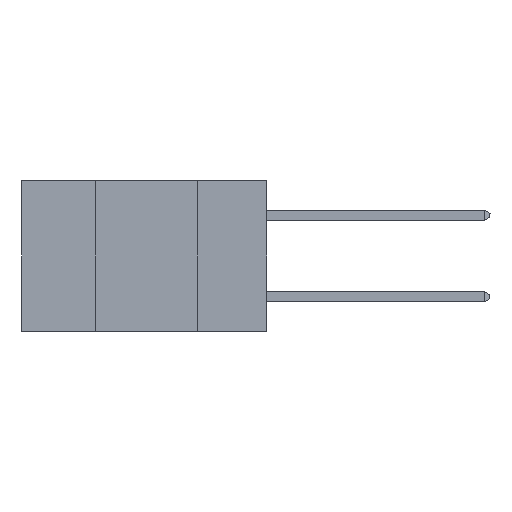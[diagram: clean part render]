
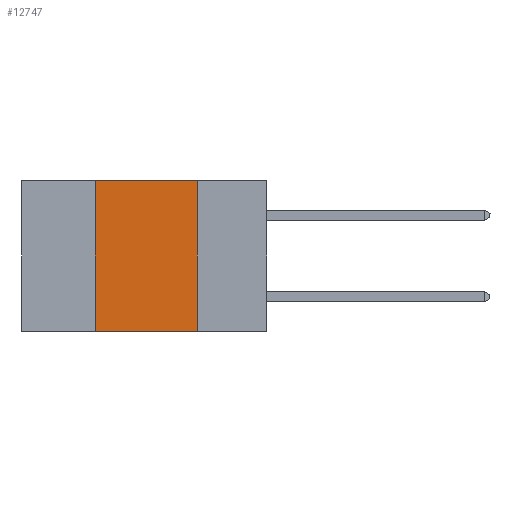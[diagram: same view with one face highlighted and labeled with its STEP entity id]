
A CAD part, left-side view. The second image highlights one B-rep face of the part: STEP entity #12747.
In plain terms, the highlighted planar face has unit normal (-1, 0, 0).
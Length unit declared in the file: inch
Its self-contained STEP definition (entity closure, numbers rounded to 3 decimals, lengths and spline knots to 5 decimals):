
#1166 = LINE ( 'NONE', #14501, #16685 ) ;
#1352 = VECTOR ( 'NONE', #8706, 39.37008 ) ;
#2403 = VECTOR ( 'NONE', #17353, 39.37008 ) ;
#2747 = CARTESIAN_POINT ( 'NONE',  ( 0., 0.17, -0.37 ) ) ;
#3363 = EDGE_CURVE ( 'NONE', #10328, #10754, #1166, .T. ) ;
#4320 = ORIENTED_EDGE ( 'NONE', *, *, #12723, .F. ) ;
#4493 = CARTESIAN_POINT ( 'NONE',  ( 0., 0.6, -0.37 ) ) ;
#5658 = ORIENTED_EDGE ( 'NONE', *, *, #3363, .F. ) ;
#6426 = LINE ( 'NONE', #15829, #2403 ) ;
#7304 = CARTESIAN_POINT ( 'NONE',  ( 0., 0.42, 0. ) ) ;
#7548 = EDGE_LOOP ( 'NONE', ( #5658, #15466, #4320, #10733 ) ) ;
#7818 = VECTOR ( 'NONE', #13415, 39.37008 ) ;
#7916 = CARTESIAN_POINT ( 'NONE',  ( 0., 0.17, 0. ) ) ;
#8090 = DIRECTION ( 'NONE',  ( 0., 0., -1. ) ) ;
#8643 = DIRECTION ( 'NONE',  ( 1., 0., 0. ) ) ;
#8706 = DIRECTION ( 'NONE',  ( 0., -1., 0. ) ) ;
#8777 = CARTESIAN_POINT ( 'NONE',  ( 0., 0.6, 0. ) ) ;
#8998 = CARTESIAN_POINT ( 'NONE',  ( 0., 0.42, -0.37 ) ) ;
#9644 = EDGE_CURVE ( 'NONE', #9987, #10754, #14302, .T. ) ;
#9987 = VERTEX_POINT ( 'NONE', #8998 ) ;
#10328 = VERTEX_POINT ( 'NONE', #7916 ) ;
#10733 = ORIENTED_EDGE ( 'NONE', *, *, #9644, .T. ) ;
#10754 = VERTEX_POINT ( 'NONE', #2747 ) ;
#11597 = FACE_OUTER_BOUND ( 'NONE', #7548, .T. ) ;
#12723 = EDGE_CURVE ( 'NONE', #9987, #15810, #6426, .T. ) ;
#12747 = ADVANCED_FACE ( 'NONE', ( #11597 ), #14829, .F. ) ;
#13415 = DIRECTION ( 'NONE',  ( 0., -1., 0. ) ) ;
#13474 = CARTESIAN_POINT ( 'NONE',  ( 0., 0.6, 0. ) ) ;
#14302 = LINE ( 'NONE', #4493, #1352 ) ;
#14501 = CARTESIAN_POINT ( 'NONE',  ( 0., 0.17, 0. ) ) ;
#14829 = PLANE ( 'NONE',  #16729 ) ;
#15466 = ORIENTED_EDGE ( 'NONE', *, *, #15719, .F. ) ;
#15719 = EDGE_CURVE ( 'NONE', #15810, #10328, #18613, .T. ) ;
#15810 = VERTEX_POINT ( 'NONE', #7304 ) ;
#15829 = CARTESIAN_POINT ( 'NONE',  ( 0., 0.42, 0. ) ) ;
#16227 = DIRECTION ( 'NONE',  ( 0., 0., -1. ) ) ;
#16685 = VECTOR ( 'NONE', #8090, 39.37008 ) ;
#16729 = AXIS2_PLACEMENT_3D ( 'NONE', #8777, #8643, #16227 ) ;
#17353 = DIRECTION ( 'NONE',  ( 0., 0., 1. ) ) ;
#18613 = LINE ( 'NONE', #13474, #7818 ) ;
